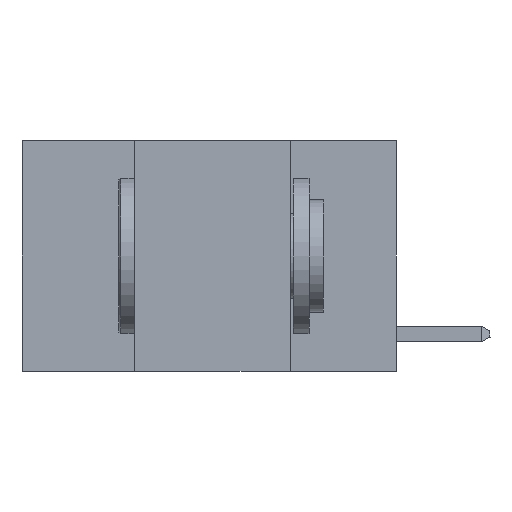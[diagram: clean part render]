
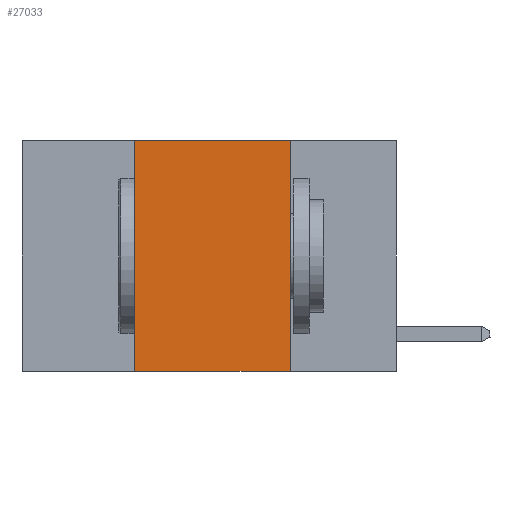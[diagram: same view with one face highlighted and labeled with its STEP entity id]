
A CAD part, left-side view. The second image highlights one B-rep face of the part: STEP entity #27033.
In plain terms, the highlighted planar face has unit normal (-1, 0, 0).
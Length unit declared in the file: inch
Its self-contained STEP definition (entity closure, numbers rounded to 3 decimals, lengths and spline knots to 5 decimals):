
#1315 = DIRECTION ( 'NONE',  ( 1., 0., 0. ) ) ;
#1414 = CARTESIAN_POINT ( 'NONE',  ( 0., 0.6, 0. ) ) ;
#2745 = ORIENTED_EDGE ( 'NONE', *, *, #26076, .T. ) ;
#3257 = EDGE_CURVE ( 'NONE', #22160, #7173, #8515, .T. ) ;
#4064 = DIRECTION ( 'NONE',  ( 0., 0., -1. ) ) ;
#4076 = CARTESIAN_POINT ( 'NONE',  ( 0., 0.42, 0. ) ) ;
#4567 = CARTESIAN_POINT ( 'NONE',  ( 0., 0.6, -0.37 ) ) ;
#5180 = EDGE_CURVE ( 'NONE', #12355, #23784, #29047, .T. ) ;
#7173 = VERTEX_POINT ( 'NONE', #9390 ) ;
#7539 = VECTOR ( 'NONE', #20673, 39.37008 ) ;
#8515 = LINE ( 'NONE', #27711, #19649 ) ;
#8558 = CARTESIAN_POINT ( 'NONE',  ( 0., 0.6, 0. ) ) ;
#9390 = CARTESIAN_POINT ( 'NONE',  ( 0., 0.17, -0.37 ) ) ;
#12355 = VERTEX_POINT ( 'NONE', #24235 ) ;
#16549 = DIRECTION ( 'NONE',  ( 0., -1., 0. ) ) ;
#16617 = VECTOR ( 'NONE', #30167, 39.37008 ) ;
#18045 = EDGE_CURVE ( 'NONE', #23784, #22160, #20923, .T. ) ;
#18122 = DIRECTION ( 'NONE',  ( 0., 0., -1. ) ) ;
#18509 = VECTOR ( 'NONE', #16549, 39.37008 ) ;
#19649 = VECTOR ( 'NONE', #4064, 39.37008 ) ;
#19980 = LINE ( 'NONE', #4567, #18509 ) ;
#20092 = CARTESIAN_POINT ( 'NONE',  ( 0., 0.17, 0. ) ) ;
#20283 = FACE_OUTER_BOUND ( 'NONE', #28965, .T. ) ;
#20673 = DIRECTION ( 'NONE',  ( 0., -1., 0. ) ) ;
#20923 = LINE ( 'NONE', #1414, #7539 ) ;
#22160 = VERTEX_POINT ( 'NONE', #20092 ) ;
#23784 = VERTEX_POINT ( 'NONE', #23906 ) ;
#23797 = ORIENTED_EDGE ( 'NONE', *, *, #5180, .F. ) ;
#23890 = ORIENTED_EDGE ( 'NONE', *, *, #18045, .F. ) ;
#23906 = CARTESIAN_POINT ( 'NONE',  ( 0., 0.42, 0. ) ) ;
#24159 = AXIS2_PLACEMENT_3D ( 'NONE', #8558, #1315, #18122 ) ;
#24235 = CARTESIAN_POINT ( 'NONE',  ( 0., 0.42, -0.37 ) ) ;
#24477 = ORIENTED_EDGE ( 'NONE', *, *, #3257, .F. ) ;
#26076 = EDGE_CURVE ( 'NONE', #12355, #7173, #19980, .T. ) ;
#27033 = ADVANCED_FACE ( 'NONE', ( #20283 ), #29768, .F. ) ;
#27711 = CARTESIAN_POINT ( 'NONE',  ( 0., 0.17, 0. ) ) ;
#28965 = EDGE_LOOP ( 'NONE', ( #24477, #23890, #23797, #2745 ) ) ;
#29047 = LINE ( 'NONE', #4076, #16617 ) ;
#29768 = PLANE ( 'NONE',  #24159 ) ;
#30167 = DIRECTION ( 'NONE',  ( 0., 0., 1. ) ) ;
